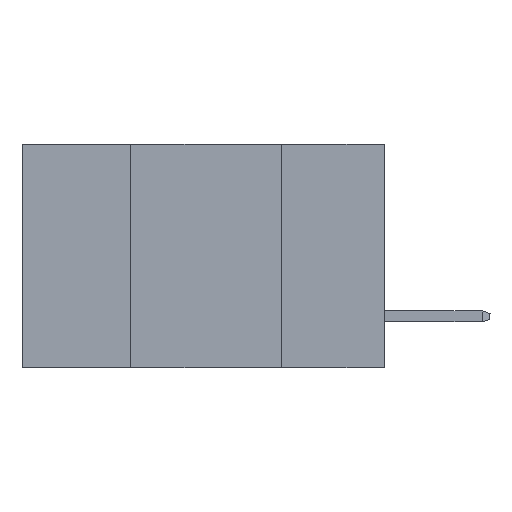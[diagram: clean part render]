
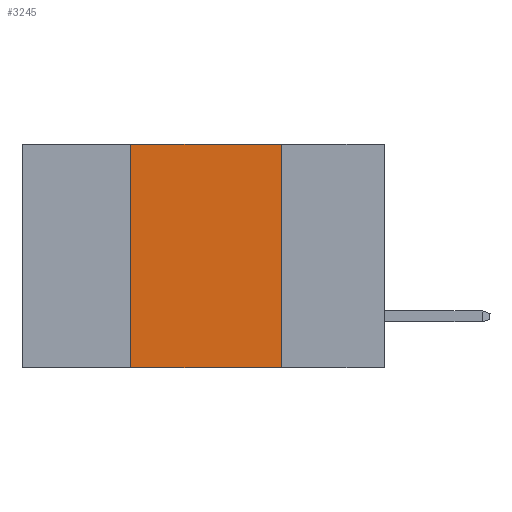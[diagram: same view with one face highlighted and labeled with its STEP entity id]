
A CAD part, left-side view. The second image highlights one B-rep face of the part: STEP entity #3245.
In plain terms, the highlighted planar face has unit normal (-1, 0, 0).
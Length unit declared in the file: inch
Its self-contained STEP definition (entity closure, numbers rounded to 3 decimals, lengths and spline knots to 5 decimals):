
#138 = EDGE_LOOP ( 'NONE', ( #15077, #16419, #957, #405 ) ) ;
#405 = ORIENTED_EDGE ( 'NONE', *, *, #13990, .T. ) ;
#957 = ORIENTED_EDGE ( 'NONE', *, *, #14108, .F. ) ;
#1259 = VECTOR ( 'NONE', #11945, 39.37008 ) ;
#1866 = DIRECTION ( 'NONE',  ( 0., 0., -1. ) ) ;
#2097 = VERTEX_POINT ( 'NONE', #14742 ) ;
#3245 = ADVANCED_FACE ( 'NONE', ( #15842 ), #9497, .F. ) ;
#3488 = CARTESIAN_POINT ( 'NONE',  ( 0., 0.6, -0.37 ) ) ;
#3983 = EDGE_CURVE ( 'NONE', #10749, #14837, #14455, .T. ) ;
#4073 = VECTOR ( 'NONE', #9840, 39.37008 ) ;
#4907 = LINE ( 'NONE', #3488, #4073 ) ;
#5526 = VERTEX_POINT ( 'NONE', #15136 ) ;
#5687 = CARTESIAN_POINT ( 'NONE',  ( 0., 0.6, 0. ) ) ;
#7652 = DIRECTION ( 'NONE',  ( 0., 0., 1. ) ) ;
#8183 = LINE ( 'NONE', #5687, #1259 ) ;
#8414 = DIRECTION ( 'NONE',  ( 0., 0., -1. ) ) ;
#9076 = EDGE_CURVE ( 'NONE', #2097, #10749, #8183, .T. ) ;
#9261 = VECTOR ( 'NONE', #1866, 39.37008 ) ;
#9414 = CARTESIAN_POINT ( 'NONE',  ( 0., 0.6, 0. ) ) ;
#9497 = PLANE ( 'NONE',  #12882 ) ;
#9840 = DIRECTION ( 'NONE',  ( 0., -1., 0. ) ) ;
#10331 = LINE ( 'NONE', #11198, #12598 ) ;
#10528 = CARTESIAN_POINT ( 'NONE',  ( 0., 0.17, -0.37 ) ) ;
#10749 = VERTEX_POINT ( 'NONE', #15343 ) ;
#11198 = CARTESIAN_POINT ( 'NONE',  ( 0., 0.42, -0.37 ) ) ;
#11945 = DIRECTION ( 'NONE',  ( 0., -1., 0. ) ) ;
#12598 = VECTOR ( 'NONE', #7652, 39.37008 ) ;
#12882 = AXIS2_PLACEMENT_3D ( 'NONE', #9414, #14501, #8414 ) ;
#13990 = EDGE_CURVE ( 'NONE', #5526, #14837, #4907, .T. ) ;
#14108 = EDGE_CURVE ( 'NONE', #5526, #2097, #10331, .T. ) ;
#14455 = LINE ( 'NONE', #15626, #9261 ) ;
#14501 = DIRECTION ( 'NONE',  ( 1., 0., 0. ) ) ;
#14742 = CARTESIAN_POINT ( 'NONE',  ( 0., 0.42, 0. ) ) ;
#14837 = VERTEX_POINT ( 'NONE', #10528 ) ;
#15077 = ORIENTED_EDGE ( 'NONE', *, *, #3983, .F. ) ;
#15136 = CARTESIAN_POINT ( 'NONE',  ( 0., 0.42, -0.37 ) ) ;
#15343 = CARTESIAN_POINT ( 'NONE',  ( 0., 0.17, 0. ) ) ;
#15626 = CARTESIAN_POINT ( 'NONE',  ( 0., 0.17, -0.37 ) ) ;
#15842 = FACE_OUTER_BOUND ( 'NONE', #138, .T. ) ;
#16419 = ORIENTED_EDGE ( 'NONE', *, *, #9076, .F. ) ;
